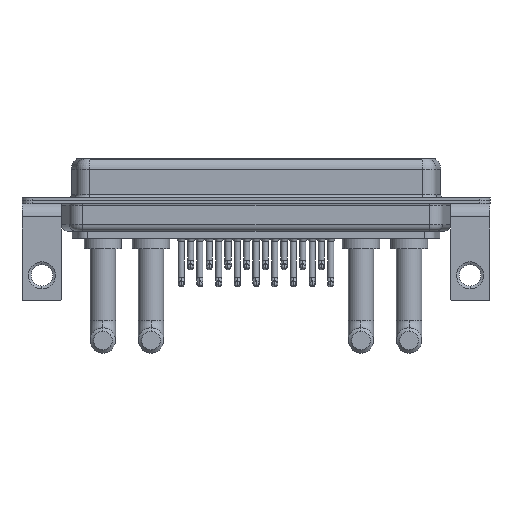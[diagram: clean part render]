
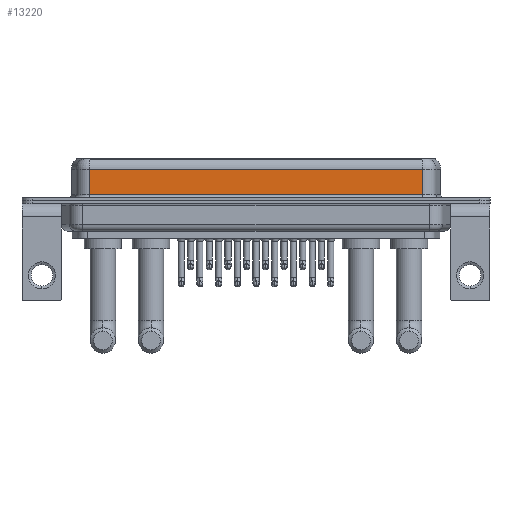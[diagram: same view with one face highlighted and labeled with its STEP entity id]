
A CAD part, front view. The second image highlights one B-rep face of the part: STEP entity #13220.
In plain terms, the highlighted planar face has unit normal (0, -1, 0).
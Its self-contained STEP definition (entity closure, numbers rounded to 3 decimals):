
#342 = ORIENTED_EDGE ( 'NONE', *, *, #6838, .F. ) ;
#775 = LINE ( 'NONE', #7816, #17688 ) ;
#1416 = LINE ( 'NONE', #15382, #22485 ) ;
#1707 = PLANE ( 'NONE',  #22155 ) ;
#1812 = CARTESIAN_POINT ( 'NONE',  ( 7.038, -3.95, 0.9 ) ) ;
#2150 = VERTEX_POINT ( 'NONE', #1812 ) ;
#2463 = ORIENTED_EDGE ( 'NONE', *, *, #3924, .T. ) ;
#3824 = CARTESIAN_POINT ( 'NONE',  ( 56.462, -3.95, 4.65 ) ) ;
#3924 = EDGE_CURVE ( 'NONE', #16508, #14243, #5171, .T. ) ;
#4511 = DIRECTION ( 'NONE',  ( 1., 0., 0. ) ) ;
#5171 = LINE ( 'NONE', #15782, #17840 ) ;
#5396 = FACE_OUTER_BOUND ( 'NONE', #11536, .T. ) ;
#6838 = EDGE_CURVE ( 'NONE', #16508, #13100, #1416, .T. ) ;
#7121 = EDGE_CURVE ( 'NONE', #2150, #13100, #11313, .T. ) ;
#7816 = CARTESIAN_POINT ( 'NONE',  ( 7.038, -3.95, 6.4 ) ) ;
#8460 = DIRECTION ( 'NONE',  ( 0., 0., -1. ) ) ;
#8530 = CARTESIAN_POINT ( 'NONE',  ( 56.462, -3.95, 6.4 ) ) ;
#8647 = DIRECTION ( 'NONE',  ( 0., 0., 1. ) ) ;
#9040 = ORIENTED_EDGE ( 'NONE', *, *, #21678, .T. ) ;
#9701 = CARTESIAN_POINT ( 'NONE',  ( 56.462, -3.95, 0.9 ) ) ;
#11313 = LINE ( 'NONE', #9701, #15937 ) ;
#11495 = DIRECTION ( 'NONE',  ( 0., 0., -1. ) ) ;
#11536 = EDGE_LOOP ( 'NONE', ( #342, #2463, #9040, #18240 ) ) ;
#12084 = DIRECTION ( 'NONE',  ( 0., 1., 0. ) ) ;
#13100 = VERTEX_POINT ( 'NONE', #22111 ) ;
#13220 = ADVANCED_FACE ( 'NONE', ( #5396 ), #1707, .F. ) ;
#14243 = VERTEX_POINT ( 'NONE', #21234 ) ;
#15382 = CARTESIAN_POINT ( 'NONE',  ( 56.462, -3.95, 6.4 ) ) ;
#15782 = CARTESIAN_POINT ( 'NONE',  ( 56.462, -3.95, 4.65 ) ) ;
#15937 = VECTOR ( 'NONE', #4511, 1000. ) ;
#16508 = VERTEX_POINT ( 'NONE', #3824 ) ;
#17688 = VECTOR ( 'NONE', #11495, 1000. ) ;
#17840 = VECTOR ( 'NONE', #18872, 1000. ) ;
#18240 = ORIENTED_EDGE ( 'NONE', *, *, #7121, .T. ) ;
#18872 = DIRECTION ( 'NONE',  ( -1., 0., 0. ) ) ;
#21234 = CARTESIAN_POINT ( 'NONE',  ( 7.038, -3.95, 4.65 ) ) ;
#21678 = EDGE_CURVE ( 'NONE', #14243, #2150, #775, .T. ) ;
#22111 = CARTESIAN_POINT ( 'NONE',  ( 56.462, -3.95, 0.9 ) ) ;
#22155 = AXIS2_PLACEMENT_3D ( 'NONE', #8530, #12084, #8647 ) ;
#22485 = VECTOR ( 'NONE', #8460, 1000. ) ;
